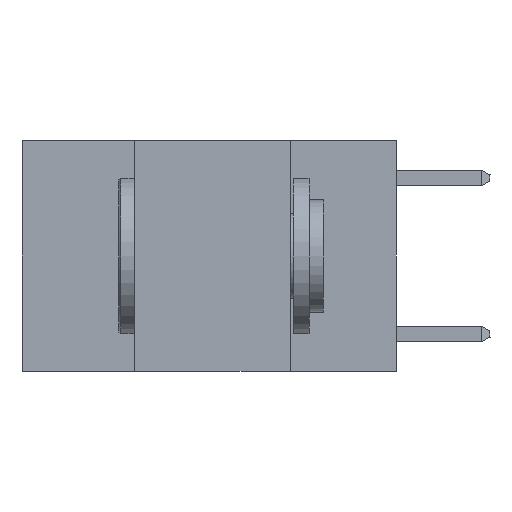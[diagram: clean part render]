
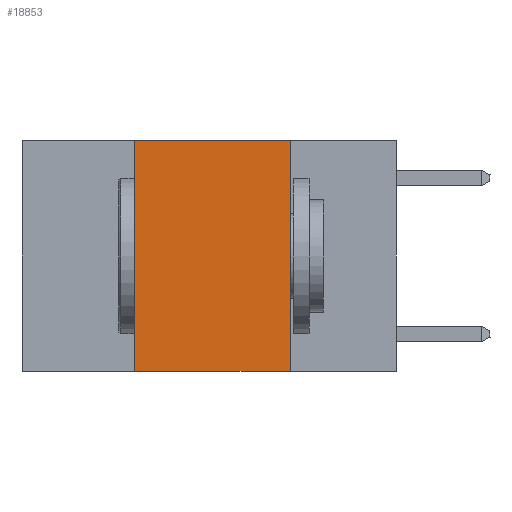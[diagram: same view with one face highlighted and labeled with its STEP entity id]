
A CAD part, left-side view. The second image highlights one B-rep face of the part: STEP entity #18853.
In plain terms, the highlighted planar face has unit normal (-1, 0, 0).
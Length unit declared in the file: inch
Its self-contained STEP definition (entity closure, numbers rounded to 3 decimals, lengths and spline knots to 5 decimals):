
#214 = EDGE_CURVE ( 'NONE', #6018, #824, #5270, .T. ) ;
#755 = LINE ( 'NONE', #3871, #13233 ) ;
#824 = VERTEX_POINT ( 'NONE', #15620 ) ;
#960 = LINE ( 'NONE', #17369, #4908 ) ;
#1087 = CARTESIAN_POINT ( 'NONE',  ( 0., 0.17, -0.37 ) ) ;
#1513 = FACE_OUTER_BOUND ( 'NONE', #19570, .T. ) ;
#2794 = CARTESIAN_POINT ( 'NONE',  ( 0., 0.6, 0. ) ) ;
#3871 = CARTESIAN_POINT ( 'NONE',  ( 0., 0.17, 0. ) ) ;
#4908 = VECTOR ( 'NONE', #8963, 39.37008 ) ;
#5247 = VECTOR ( 'NONE', #16393, 39.37008 ) ;
#5270 = LINE ( 'NONE', #13141, #5247 ) ;
#5475 = EDGE_CURVE ( 'NONE', #14857, #6018, #20816, .T. ) ;
#5518 = DIRECTION ( 'NONE',  ( 0., 0., -1. ) ) ;
#5603 = ORIENTED_EDGE ( 'NONE', *, *, #17939, .F. ) ;
#5989 = ORIENTED_EDGE ( 'NONE', *, *, #214, .F. ) ;
#6018 = VERTEX_POINT ( 'NONE', #14472 ) ;
#6073 = ORIENTED_EDGE ( 'NONE', *, *, #5475, .F. ) ;
#6322 = ORIENTED_EDGE ( 'NONE', *, *, #6601, .T. ) ;
#6601 = EDGE_CURVE ( 'NONE', #14857, #16988, #960, .T. ) ;
#7869 = PLANE ( 'NONE',  #17171 ) ;
#8963 = DIRECTION ( 'NONE',  ( 0., -1., 0. ) ) ;
#9620 = DIRECTION ( 'NONE',  ( 1., 0., 0. ) ) ;
#13141 = CARTESIAN_POINT ( 'NONE',  ( 0., 0.6, 0. ) ) ;
#13233 = VECTOR ( 'NONE', #5518, 39.37008 ) ;
#14472 = CARTESIAN_POINT ( 'NONE',  ( 0., 0.42, 0. ) ) ;
#14857 = VERTEX_POINT ( 'NONE', #20940 ) ;
#15620 = CARTESIAN_POINT ( 'NONE',  ( 0., 0.17, 0. ) ) ;
#16393 = DIRECTION ( 'NONE',  ( 0., -1., 0. ) ) ;
#16624 = VECTOR ( 'NONE', #21142, 39.37008 ) ;
#16988 = VERTEX_POINT ( 'NONE', #1087 ) ;
#17171 = AXIS2_PLACEMENT_3D ( 'NONE', #2794, #9620, #21079 ) ;
#17369 = CARTESIAN_POINT ( 'NONE',  ( 0., 0.6, -0.37 ) ) ;
#17939 = EDGE_CURVE ( 'NONE', #824, #16988, #755, .T. ) ;
#18032 = CARTESIAN_POINT ( 'NONE',  ( 0., 0.42, 0. ) ) ;
#18853 = ADVANCED_FACE ( 'NONE', ( #1513 ), #7869, .F. ) ;
#19570 = EDGE_LOOP ( 'NONE', ( #5603, #5989, #6073, #6322 ) ) ;
#20816 = LINE ( 'NONE', #18032, #16624 ) ;
#20940 = CARTESIAN_POINT ( 'NONE',  ( 0., 0.42, -0.37 ) ) ;
#21079 = DIRECTION ( 'NONE',  ( 0., 0., -1. ) ) ;
#21142 = DIRECTION ( 'NONE',  ( 0., 0., 1. ) ) ;
